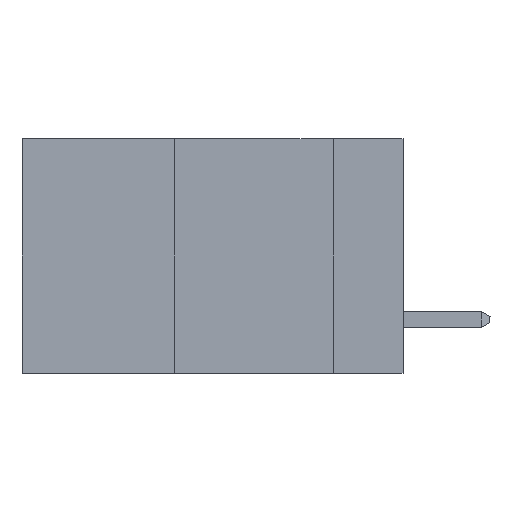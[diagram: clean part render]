
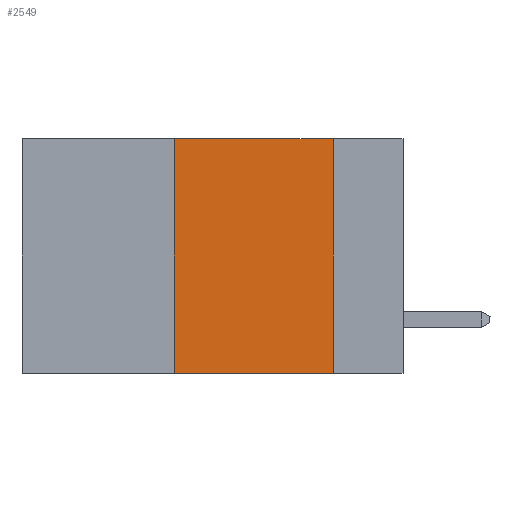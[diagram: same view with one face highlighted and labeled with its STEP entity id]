
A CAD part, left-side view. The second image highlights one B-rep face of the part: STEP entity #2549.
In plain terms, the highlighted planar face has unit normal (-1, 0, 0).
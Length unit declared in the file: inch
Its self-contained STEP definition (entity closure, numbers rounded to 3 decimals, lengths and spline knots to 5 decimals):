
#1010 = EDGE_LOOP ( 'NONE', ( #21159, #10902, #16119, #13017 ) ) ;
#1118 = CARTESIAN_POINT ( 'NONE',  ( 0., 0.6, 0. ) ) ;
#1566 = FACE_OUTER_BOUND ( 'NONE', #1010, .T. ) ;
#2509 = VECTOR ( 'NONE', #9470, 39.37008 ) ;
#2549 = ADVANCED_FACE ( 'NONE', ( #1566 ), #15334, .F. ) ;
#2803 = DIRECTION ( 'NONE',  ( 0., 0., -1. ) ) ;
#3480 = LINE ( 'NONE', #10379, #8091 ) ;
#3793 = EDGE_CURVE ( 'NONE', #12964, #15868, #3480, .T. ) ;
#5858 = LINE ( 'NONE', #9246, #2509 ) ;
#6201 = DIRECTION ( 'NONE',  ( 1., 0., 0. ) ) ;
#6585 = CARTESIAN_POINT ( 'NONE',  ( 0., 0.11, 0. ) ) ;
#7520 = VECTOR ( 'NONE', #18971, 39.37008 ) ;
#7822 = CARTESIAN_POINT ( 'NONE',  ( 0., 0.36, -0.37 ) ) ;
#8066 = VERTEX_POINT ( 'NONE', #7822 ) ;
#8091 = VECTOR ( 'NONE', #14959, 39.37008 ) ;
#9147 = CARTESIAN_POINT ( 'NONE',  ( 0., 0.36, 0. ) ) ;
#9246 = CARTESIAN_POINT ( 'NONE',  ( 0., 0.36, 0. ) ) ;
#9470 = DIRECTION ( 'NONE',  ( 0., 0., 1. ) ) ;
#10013 = CARTESIAN_POINT ( 'NONE',  ( 0., 0.6, -0.37 ) ) ;
#10346 = LINE ( 'NONE', #10013, #15784 ) ;
#10379 = CARTESIAN_POINT ( 'NONE',  ( 0., 0.11, 0. ) ) ;
#10519 = CARTESIAN_POINT ( 'NONE',  ( 0., 0.6, 0. ) ) ;
#10902 = ORIENTED_EDGE ( 'NONE', *, *, #18472, .F. ) ;
#12964 = VERTEX_POINT ( 'NONE', #6585 ) ;
#13017 = ORIENTED_EDGE ( 'NONE', *, *, #17981, .T. ) ;
#13406 = DIRECTION ( 'NONE',  ( 0., -1., 0. ) ) ;
#14007 = LINE ( 'NONE', #10519, #7520 ) ;
#14690 = CARTESIAN_POINT ( 'NONE',  ( 0., 0.11, -0.37 ) ) ;
#14959 = DIRECTION ( 'NONE',  ( 0., 0., -1. ) ) ;
#15334 = PLANE ( 'NONE',  #19093 ) ;
#15784 = VECTOR ( 'NONE', #13406, 39.37008 ) ;
#15868 = VERTEX_POINT ( 'NONE', #14690 ) ;
#16119 = ORIENTED_EDGE ( 'NONE', *, *, #20946, .F. ) ;
#17340 = VERTEX_POINT ( 'NONE', #9147 ) ;
#17981 = EDGE_CURVE ( 'NONE', #8066, #15868, #10346, .T. ) ;
#18472 = EDGE_CURVE ( 'NONE', #17340, #12964, #14007, .T. ) ;
#18971 = DIRECTION ( 'NONE',  ( 0., -1., 0. ) ) ;
#19093 = AXIS2_PLACEMENT_3D ( 'NONE', #1118, #6201, #2803 ) ;
#20946 = EDGE_CURVE ( 'NONE', #8066, #17340, #5858, .T. ) ;
#21159 = ORIENTED_EDGE ( 'NONE', *, *, #3793, .F. ) ;
